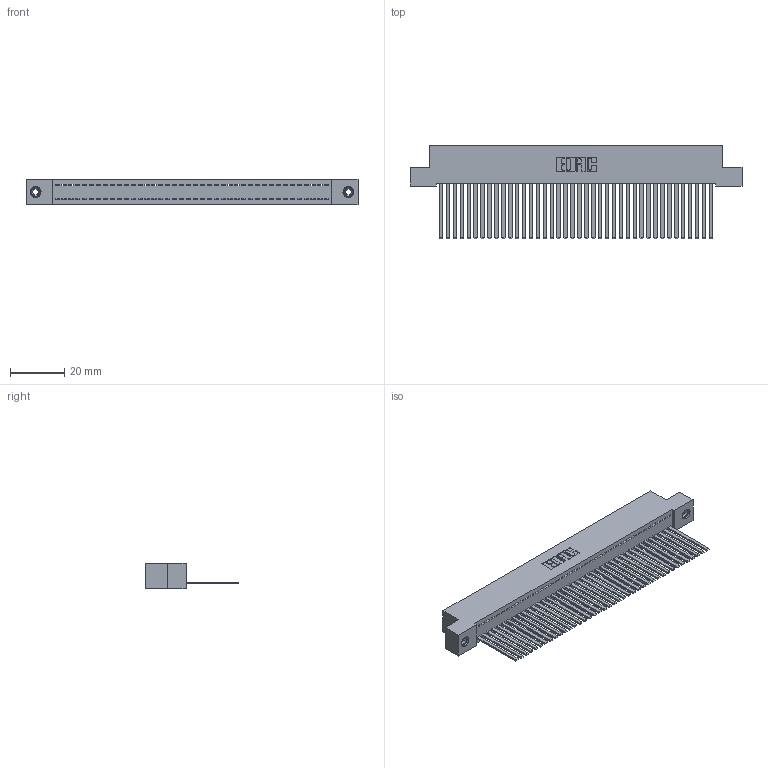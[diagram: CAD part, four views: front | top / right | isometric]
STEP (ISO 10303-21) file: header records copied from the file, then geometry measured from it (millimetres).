
FILE_DESCRIPTION (( 'STEP AP203' ), '1' );
FILE_NAME ('392-040-544-108.STEP', '2018-08-16T12:21:08', ( '' ), ( '' ), 'SwSTEP 2.0', 'SolidWorks 2016', '' );
FILE_SCHEMA (( 'CONFIG_CONTROL_DESIGN' ));
Length unit declared in the file: inch
Products named in the file (4): 342 Part_TI; 345-292-001_345-293-144; 345-250-001_345-250-003-102; 392-040-544-108
Assembly tree (43 placements, depth 2):
  392-040-544-108
    342 Part_TI
    345-292-001_345-293-144  x40
    345-250-001_345-250-003-102  x2
Bounding box: 121.92 x 34.3 x 9.4 mm (x, y, z)
Volume: 11140.1 mm3; surface area: 17657.7 mm2
Topology: 43 solids, 43 shells, 2250 faces, 6755 edges, 4442 vertices
Faces by surface type: plane 1618, cylinder 616, cone 12, torus 4
Entity records: 25582 total; most frequent: CARTESIAN_POINT 4393, ORIENTED_EDGE 4362, DIRECTION 3739, EDGE_CURVE 2181, LINE 2037, VECTOR 2037, VERTEX_POINT 1448, AXIS2_PLACEMENT_3D 851
